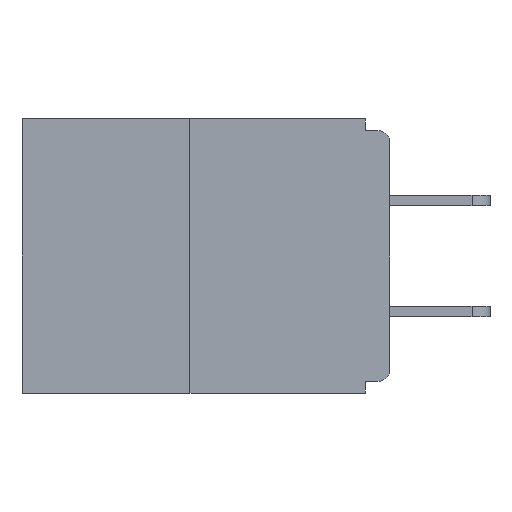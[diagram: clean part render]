
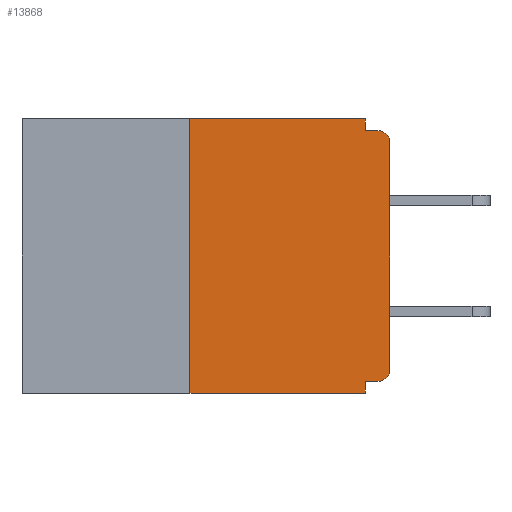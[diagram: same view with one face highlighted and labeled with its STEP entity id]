
A CAD part, left-side view. The second image highlights one B-rep face of the part: STEP entity #13868.
In plain terms, the highlighted planar face has unit normal (-1, 0, 0).
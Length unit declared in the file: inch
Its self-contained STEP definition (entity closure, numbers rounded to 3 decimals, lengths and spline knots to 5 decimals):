
#154 = AXIS2_PLACEMENT_3D ( 'NONE', #337, #1942, #2410 ) ;
#195 = EDGE_CURVE ( 'NONE', #4076, #453, #3492, .T. ) ;
#337 = CARTESIAN_POINT ( 'NONE',  ( 0., 0.015, -0.313 ) ) ;
#453 = VERTEX_POINT ( 'NONE', #6733 ) ;
#687 = CARTESIAN_POINT ( 'NONE',  ( 0., 0.25, -0.343 ) ) ;
#733 = EDGE_CURVE ( 'NONE', #9544, #12976, #4194, .T. ) ;
#780 = CARTESIAN_POINT ( 'NONE',  ( 0., 0., -0.015 ) ) ;
#1050 = DIRECTION ( 'NONE',  ( 0., -1., 0. ) ) ;
#1189 = VECTOR ( 'NONE', #11210, 39.37008 ) ;
#1786 = DIRECTION ( 'NONE',  ( 0., 0., 1. ) ) ;
#1942 = DIRECTION ( 'NONE',  ( -1., 0., 0. ) ) ;
#2011 = DIRECTION ( 'NONE',  ( -1., 0., 0. ) ) ;
#2293 = CARTESIAN_POINT ( 'NONE',  ( 0., 0.25, 0. ) ) ;
#2410 = DIRECTION ( 'NONE',  ( 0., 0., -1. ) ) ;
#2905 = DIRECTION ( 'NONE',  ( 0., 1., 0. ) ) ;
#2975 = CARTESIAN_POINT ( 'NONE',  ( 0., 0., -0.328 ) ) ;
#3492 = CIRCLE ( 'NONE', #7655, 0.015 ) ;
#3504 = CARTESIAN_POINT ( 'NONE',  ( 0., 0., -0.313 ) ) ;
#4076 = VERTEX_POINT ( 'NONE', #18809 ) ;
#4182 = EDGE_CURVE ( 'NONE', #17657, #453, #11340, .T. ) ;
#4194 = LINE ( 'NONE', #17692, #8216 ) ;
#4443 = CARTESIAN_POINT ( 'NONE',  ( 0., 0.031, 0. ) ) ;
#4549 = FACE_OUTER_BOUND ( 'NONE', #13998, .T. ) ;
#4985 = ORIENTED_EDGE ( 'NONE', *, *, #7807, .F. ) ;
#5072 = LINE ( 'NONE', #18473, #7897 ) ;
#5448 = CARTESIAN_POINT ( 'NONE',  ( 0., 0.031, -0.015 ) ) ;
#5549 = CARTESIAN_POINT ( 'NONE',  ( 0., 0.031, -0.343 ) ) ;
#5693 = ORIENTED_EDGE ( 'NONE', *, *, #733, .F. ) ;
#6337 = VERTEX_POINT ( 'NONE', #15402 ) ;
#6733 = CARTESIAN_POINT ( 'NONE',  ( 0., 0.015, -0.015 ) ) ;
#6933 = EDGE_CURVE ( 'NONE', #11011, #14373, #6973, .T. ) ;
#6973 = CIRCLE ( 'NONE', #154, 0.015 ) ;
#7078 = DIRECTION ( 'NONE',  ( 0., -1., 0. ) ) ;
#7485 = EDGE_CURVE ( 'NONE', #16264, #6337, #19069, .T. ) ;
#7655 = AXIS2_PLACEMENT_3D ( 'NONE', #10832, #2011, #13984 ) ;
#7807 = EDGE_CURVE ( 'NONE', #12976, #17657, #10930, .T. ) ;
#7897 = VECTOR ( 'NONE', #1786, 39.37008 ) ;
#8145 = LINE ( 'NONE', #16389, #10051 ) ;
#8216 = VECTOR ( 'NONE', #1050, 39.37008 ) ;
#8762 = DIRECTION ( 'NONE',  ( 0., 0., -1. ) ) ;
#9470 = VECTOR ( 'NONE', #8762, 39.37008 ) ;
#9544 = VERTEX_POINT ( 'NONE', #2293 ) ;
#10051 = VECTOR ( 'NONE', #17927, 39.37008 ) ;
#10140 = ORIENTED_EDGE ( 'NONE', *, *, #195, .T. ) ;
#10421 = DIRECTION ( 'NONE',  ( 0., 0., -1. ) ) ;
#10832 = CARTESIAN_POINT ( 'NONE',  ( 0., 0.015, -0.03 ) ) ;
#10841 = ORIENTED_EDGE ( 'NONE', *, *, #15168, .F. ) ;
#10930 = LINE ( 'NONE', #4443, #19277 ) ;
#11011 = VERTEX_POINT ( 'NONE', #15169 ) ;
#11210 = DIRECTION ( 'NONE',  ( 0., -1., 0. ) ) ;
#11340 = LINE ( 'NONE', #780, #1189 ) ;
#11869 = VECTOR ( 'NONE', #2905, 39.37008 ) ;
#11920 = ORIENTED_EDGE ( 'NONE', *, *, #19105, .F. ) ;
#12478 = EDGE_CURVE ( 'NONE', #14373, #4076, #5072, .T. ) ;
#12976 = VERTEX_POINT ( 'NONE', #14663 ) ;
#13186 = ORIENTED_EDGE ( 'NONE', *, *, #7485, .T. ) ;
#13250 = ORIENTED_EDGE ( 'NONE', *, *, #4182, .F. ) ;
#13304 = CARTESIAN_POINT ( 'NONE',  ( 0., 0.46, 0. ) ) ;
#13868 = ADVANCED_FACE ( 'NONE', ( #4549 ), #16349, .F. ) ;
#13984 = DIRECTION ( 'NONE',  ( 0., 0., -1. ) ) ;
#13998 = EDGE_LOOP ( 'NONE', ( #5693, #11920, #13186, #10841, #15475, #17928, #18231, #10140, #13250, #4985 ) ) ;
#14079 = VECTOR ( 'NONE', #7078, 39.37008 ) ;
#14142 = AXIS2_PLACEMENT_3D ( 'NONE', #13304, #16285, #10421 ) ;
#14373 = VERTEX_POINT ( 'NONE', #3504 ) ;
#14663 = CARTESIAN_POINT ( 'NONE',  ( 0., 0.031, 0. ) ) ;
#14803 = EDGE_CURVE ( 'NONE', #11011, #17376, #18069, .T. ) ;
#15039 = DIRECTION ( 'NONE',  ( 0., 0., -1. ) ) ;
#15168 = EDGE_CURVE ( 'NONE', #17376, #6337, #19006, .T. ) ;
#15169 = CARTESIAN_POINT ( 'NONE',  ( 0., 0.015, -0.328 ) ) ;
#15402 = CARTESIAN_POINT ( 'NONE',  ( 0., 0.031, -0.343 ) ) ;
#15475 = ORIENTED_EDGE ( 'NONE', *, *, #14803, .F. ) ;
#16034 = CARTESIAN_POINT ( 'NONE',  ( 0., 0.46, -0.343 ) ) ;
#16264 = VERTEX_POINT ( 'NONE', #687 ) ;
#16285 = DIRECTION ( 'NONE',  ( 1., 0., 0. ) ) ;
#16349 = PLANE ( 'NONE',  #14142 ) ;
#16389 = CARTESIAN_POINT ( 'NONE',  ( 0., 0.25, 0. ) ) ;
#17376 = VERTEX_POINT ( 'NONE', #17931 ) ;
#17657 = VERTEX_POINT ( 'NONE', #5448 ) ;
#17692 = CARTESIAN_POINT ( 'NONE',  ( 0., 0.46, 0. ) ) ;
#17927 = DIRECTION ( 'NONE',  ( 0., 0., 1. ) ) ;
#17928 = ORIENTED_EDGE ( 'NONE', *, *, #6933, .T. ) ;
#17931 = CARTESIAN_POINT ( 'NONE',  ( 0., 0.031, -0.328 ) ) ;
#18069 = LINE ( 'NONE', #2975, #11869 ) ;
#18231 = ORIENTED_EDGE ( 'NONE', *, *, #12478, .T. ) ;
#18473 = CARTESIAN_POINT ( 'NONE',  ( 0., 0., 0. ) ) ;
#18809 = CARTESIAN_POINT ( 'NONE',  ( 0., 0., -0.03 ) ) ;
#19006 = LINE ( 'NONE', #5549, #9470 ) ;
#19069 = LINE ( 'NONE', #16034, #14079 ) ;
#19105 = EDGE_CURVE ( 'NONE', #16264, #9544, #8145, .T. ) ;
#19277 = VECTOR ( 'NONE', #15039, 39.37008 ) ;
